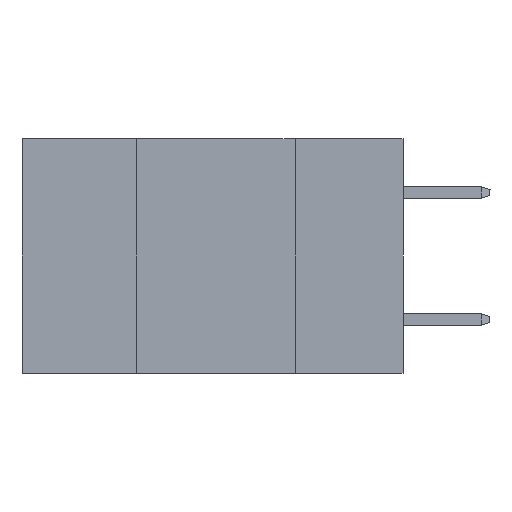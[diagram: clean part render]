
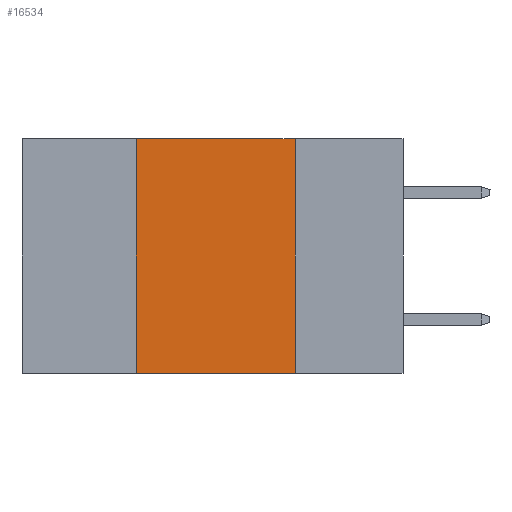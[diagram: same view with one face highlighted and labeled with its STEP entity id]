
A CAD part, left-side view. The second image highlights one B-rep face of the part: STEP entity #16534.
In plain terms, the highlighted planar face has unit normal (-1, 0, 0).
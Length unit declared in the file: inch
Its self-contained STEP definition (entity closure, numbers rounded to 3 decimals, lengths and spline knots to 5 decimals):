
#440 = EDGE_LOOP ( 'NONE', ( #14234, #19335, #6127, #6750 ) ) ;
#775 = VECTOR ( 'NONE', #17072, 39.37008 ) ;
#1358 = VERTEX_POINT ( 'NONE', #5999 ) ;
#1985 = FACE_OUTER_BOUND ( 'NONE', #440, .T. ) ;
#2269 = CARTESIAN_POINT ( 'NONE',  ( 0., 0.6, -0.37 ) ) ;
#2855 = DIRECTION ( 'NONE',  ( 0., -1., 0. ) ) ;
#3641 = DIRECTION ( 'NONE',  ( 1., 0., 0. ) ) ;
#5999 = CARTESIAN_POINT ( 'NONE',  ( 0., 0.17, -0.37 ) ) ;
#6127 = ORIENTED_EDGE ( 'NONE', *, *, #11255, .F. ) ;
#6750 = ORIENTED_EDGE ( 'NONE', *, *, #18431, .T. ) ;
#6828 = PLANE ( 'NONE',  #15801 ) ;
#7739 = CARTESIAN_POINT ( 'NONE',  ( 0., 0.42, -0.37 ) ) ;
#9966 = DIRECTION ( 'NONE',  ( 0., 0., 1. ) ) ;
#10402 = VERTEX_POINT ( 'NONE', #13422 ) ;
#10425 = DIRECTION ( 'NONE',  ( 0., -1., 0. ) ) ;
#10857 = LINE ( 'NONE', #18814, #775 ) ;
#11255 = EDGE_CURVE ( 'NONE', #12043, #10402, #19320, .T. ) ;
#11503 = VECTOR ( 'NONE', #2855, 39.37008 ) ;
#12043 = VERTEX_POINT ( 'NONE', #7739 ) ;
#12763 = CARTESIAN_POINT ( 'NONE',  ( 0., 0.17, 0. ) ) ;
#13091 = DIRECTION ( 'NONE',  ( 0., 0., -1. ) ) ;
#13422 = CARTESIAN_POINT ( 'NONE',  ( 0., 0.42, 0. ) ) ;
#13505 = VECTOR ( 'NONE', #10425, 39.37008 ) ;
#14234 = ORIENTED_EDGE ( 'NONE', *, *, #18237, .F. ) ;
#14415 = EDGE_CURVE ( 'NONE', #10402, #15561, #16701, .T. ) ;
#14531 = CARTESIAN_POINT ( 'NONE',  ( 0., 0.6, 0. ) ) ;
#15561 = VERTEX_POINT ( 'NONE', #12763 ) ;
#15801 = AXIS2_PLACEMENT_3D ( 'NONE', #14531, #3641, #13091 ) ;
#16534 = ADVANCED_FACE ( 'NONE', ( #1985 ), #6828, .F. ) ;
#16701 = LINE ( 'NONE', #18234, #11503 ) ;
#17072 = DIRECTION ( 'NONE',  ( 0., 0., -1. ) ) ;
#17792 = CARTESIAN_POINT ( 'NONE',  ( 0., 0.42, 0. ) ) ;
#18234 = CARTESIAN_POINT ( 'NONE',  ( 0., 0.6, 0. ) ) ;
#18237 = EDGE_CURVE ( 'NONE', #15561, #1358, #10857, .T. ) ;
#18363 = VECTOR ( 'NONE', #9966, 39.37008 ) ;
#18431 = EDGE_CURVE ( 'NONE', #12043, #1358, #19797, .T. ) ;
#18814 = CARTESIAN_POINT ( 'NONE',  ( 0., 0.17, 0. ) ) ;
#19320 = LINE ( 'NONE', #17792, #18363 ) ;
#19335 = ORIENTED_EDGE ( 'NONE', *, *, #14415, .F. ) ;
#19797 = LINE ( 'NONE', #2269, #13505 ) ;
